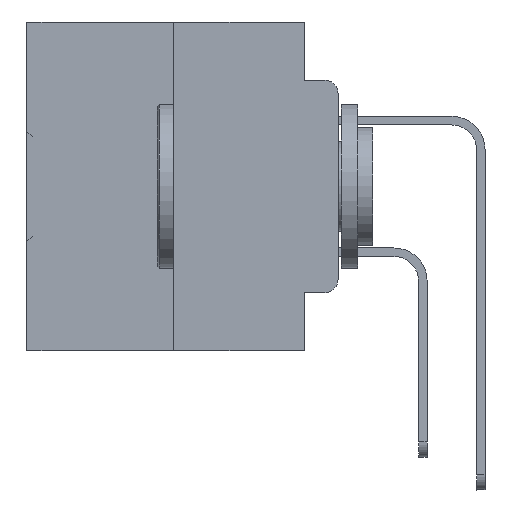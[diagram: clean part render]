
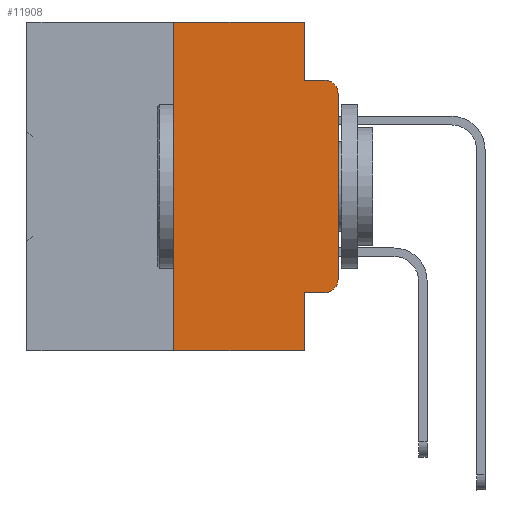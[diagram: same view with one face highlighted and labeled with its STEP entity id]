
A CAD part, left-side view. The second image highlights one B-rep face of the part: STEP entity #11908.
In plain terms, the highlighted planar face has unit normal (-1, 0, 0).
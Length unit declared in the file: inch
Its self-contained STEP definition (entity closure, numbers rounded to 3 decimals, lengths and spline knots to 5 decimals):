
#683 = EDGE_CURVE ( 'NONE', #8912, #12621, #1866, .T. ) ;
#1227 = CARTESIAN_POINT ( 'NONE',  ( 0., 0.051, -0.4115 ) ) ;
#1825 = DIRECTION ( 'NONE',  ( 0., 0., 1. ) ) ;
#1866 = LINE ( 'NONE', #27955, #32161 ) ;
#1879 = AXIS2_PLACEMENT_3D ( 'NONE', #7233, #22005, #4373 ) ;
#1899 = CARTESIAN_POINT ( 'NONE',  ( 0., 0., -0.3915 ) ) ;
#2024 = LINE ( 'NONE', #36897, #9879 ) ;
#2343 = ORIENTED_EDGE ( 'NONE', *, *, #6626, .F. ) ;
#2837 = AXIS2_PLACEMENT_3D ( 'NONE', #15590, #36089, #18597 ) ;
#2909 = EDGE_CURVE ( 'NONE', #5547, #16486, #24207, .T. ) ;
#3063 = LINE ( 'NONE', #21507, #18740 ) ;
#3302 = CARTESIAN_POINT ( 'NONE',  ( 0., 0.473, -0.5 ) ) ;
#3533 = CARTESIAN_POINT ( 'NONE',  ( 0., 0.051, -0.0885 ) ) ;
#3702 = ORIENTED_EDGE ( 'NONE', *, *, #2909, .F. ) ;
#3740 = ORIENTED_EDGE ( 'NONE', *, *, #36750, .T. ) ;
#4373 = DIRECTION ( 'NONE',  ( 0., 0., -1. ) ) ;
#5120 = EDGE_CURVE ( 'NONE', #13659, #12621, #29124, .T. ) ;
#5547 = VERTEX_POINT ( 'NONE', #29756 ) ;
#6626 = EDGE_CURVE ( 'NONE', #13659, #5547, #2024, .T. ) ;
#6738 = CARTESIAN_POINT ( 'NONE',  ( 0., 0.25, -0.5 ) ) ;
#7233 = CARTESIAN_POINT ( 'NONE',  ( 0., 0.473, 0. ) ) ;
#7641 = CIRCLE ( 'NONE', #33501, 0.02 ) ;
#8605 = EDGE_CURVE ( 'NONE', #16486, #19164, #35856, .T. ) ;
#8912 = VERTEX_POINT ( 'NONE', #1227 ) ;
#9536 = VECTOR ( 'NONE', #19150, 39.37008 ) ;
#9879 = VECTOR ( 'NONE', #1825, 39.37008 ) ;
#10518 = DIRECTION ( 'NONE',  ( -1., 0., 0. ) ) ;
#10559 = EDGE_CURVE ( 'NONE', #19164, #30876, #37932, .T. ) ;
#11566 = ORIENTED_EDGE ( 'NONE', *, *, #32901, .T. ) ;
#11908 = ADVANCED_FACE ( 'NONE', ( #30141 ), #19041, .F. ) ;
#12441 = CARTESIAN_POINT ( 'NONE',  ( 0., 0.02, -0.4115 ) ) ;
#12460 = ORIENTED_EDGE ( 'NONE', *, *, #20396, .T. ) ;
#12621 = VERTEX_POINT ( 'NONE', #25651 ) ;
#13659 = VERTEX_POINT ( 'NONE', #6738 ) ;
#13727 = CARTESIAN_POINT ( 'NONE',  ( 0., 0., 0. ) ) ;
#14221 = VERTEX_POINT ( 'NONE', #12441 ) ;
#14340 = VECTOR ( 'NONE', #19684, 39.37008 ) ;
#14612 = VECTOR ( 'NONE', #29986, 39.37008 ) ;
#15590 = CARTESIAN_POINT ( 'NONE',  ( 0., 0.02, -0.3915 ) ) ;
#16261 = EDGE_LOOP ( 'NONE', ( #12460, #23918, #17933, #17477, #3702, #2343, #17972, #35383, #3740, #11566 ) ) ;
#16399 = EDGE_CURVE ( 'NONE', #29807, #30876, #7641, .T. ) ;
#16486 = VERTEX_POINT ( 'NONE', #22565 ) ;
#17372 = CARTESIAN_POINT ( 'NONE',  ( 0., 0.473, 0. ) ) ;
#17477 = ORIENTED_EDGE ( 'NONE', *, *, #8605, .F. ) ;
#17933 = ORIENTED_EDGE ( 'NONE', *, *, #10559, .F. ) ;
#17972 = ORIENTED_EDGE ( 'NONE', *, *, #5120, .T. ) ;
#18401 = CARTESIAN_POINT ( 'NONE',  ( 0., 0., -0.1085 ) ) ;
#18597 = DIRECTION ( 'NONE',  ( 0., 0., -1. ) ) ;
#18740 = VECTOR ( 'NONE', #24427, 39.37008 ) ;
#19041 = PLANE ( 'NONE',  #1879 ) ;
#19150 = DIRECTION ( 'NONE',  ( 0., -1., 0. ) ) ;
#19164 = VERTEX_POINT ( 'NONE', #19527 ) ;
#19527 = CARTESIAN_POINT ( 'NONE',  ( 0., 0.051, -0.0885 ) ) ;
#19684 = DIRECTION ( 'NONE',  ( 0., 0., 1. ) ) ;
#20334 = VECTOR ( 'NONE', #20532, 39.37008 ) ;
#20363 = LINE ( 'NONE', #13727, #14340 ) ;
#20396 = EDGE_CURVE ( 'NONE', #22854, #29807, #20363, .T. ) ;
#20435 = VECTOR ( 'NONE', #33359, 39.37008 ) ;
#20532 = DIRECTION ( 'NONE',  ( 0., 0., -1. ) ) ;
#21507 = CARTESIAN_POINT ( 'NONE',  ( 0., 0.051, -0.4115 ) ) ;
#22005 = DIRECTION ( 'NONE',  ( 1., 0., 0. ) ) ;
#22276 = CIRCLE ( 'NONE', #2837, 0.02 ) ;
#22565 = CARTESIAN_POINT ( 'NONE',  ( 0., 0.051, 0. ) ) ;
#22854 = VERTEX_POINT ( 'NONE', #1899 ) ;
#23918 = ORIENTED_EDGE ( 'NONE', *, *, #16399, .T. ) ;
#24207 = LINE ( 'NONE', #17372, #9536 ) ;
#24427 = DIRECTION ( 'NONE',  ( 0., -1., 0. ) ) ;
#25651 = CARTESIAN_POINT ( 'NONE',  ( 0., 0.051, -0.5 ) ) ;
#26156 = DIRECTION ( 'NONE',  ( 0., 0., -1. ) ) ;
#27955 = CARTESIAN_POINT ( 'NONE',  ( 0., 0.051, 0. ) ) ;
#28096 = CARTESIAN_POINT ( 'NONE',  ( 0., 0.02, -0.1085 ) ) ;
#29079 = CARTESIAN_POINT ( 'NONE',  ( 0., 0.02, -0.0885 ) ) ;
#29124 = LINE ( 'NONE', #3302, #20435 ) ;
#29229 = CARTESIAN_POINT ( 'NONE',  ( 0., 0.051, 0. ) ) ;
#29756 = CARTESIAN_POINT ( 'NONE',  ( 0., 0.25, 0. ) ) ;
#29807 = VERTEX_POINT ( 'NONE', #18401 ) ;
#29986 = DIRECTION ( 'NONE',  ( 0., -1., 0. ) ) ;
#30141 = FACE_OUTER_BOUND ( 'NONE', #16261, .T. ) ;
#30876 = VERTEX_POINT ( 'NONE', #29079 ) ;
#31010 = DIRECTION ( 'NONE',  ( 0., 0., -1. ) ) ;
#32161 = VECTOR ( 'NONE', #26156, 39.37008 ) ;
#32901 = EDGE_CURVE ( 'NONE', #14221, #22854, #22276, .T. ) ;
#33359 = DIRECTION ( 'NONE',  ( 0., -1., 0. ) ) ;
#33501 = AXIS2_PLACEMENT_3D ( 'NONE', #28096, #10518, #31010 ) ;
#35383 = ORIENTED_EDGE ( 'NONE', *, *, #683, .F. ) ;
#35856 = LINE ( 'NONE', #29229, #20334 ) ;
#36089 = DIRECTION ( 'NONE',  ( -1., 0., 0. ) ) ;
#36750 = EDGE_CURVE ( 'NONE', #8912, #14221, #3063, .T. ) ;
#36897 = CARTESIAN_POINT ( 'NONE',  ( 0., 0.25, 0. ) ) ;
#37932 = LINE ( 'NONE', #3533, #14612 ) ;
